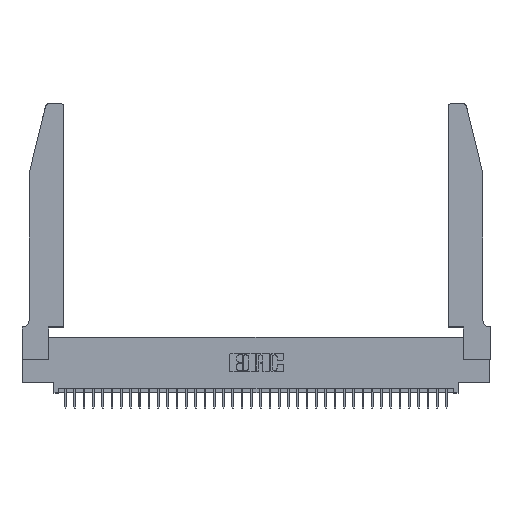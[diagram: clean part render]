
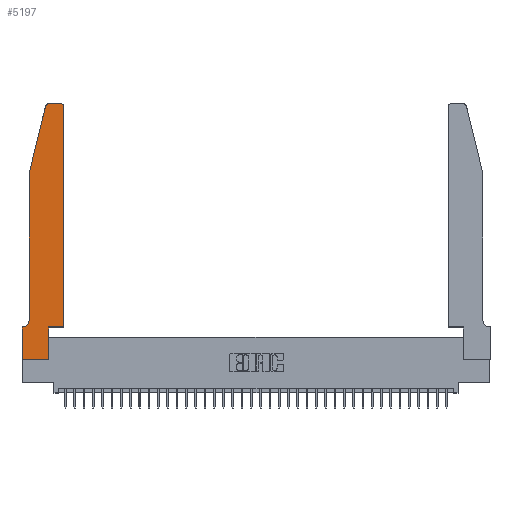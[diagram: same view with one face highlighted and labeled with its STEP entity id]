
A CAD part, top view. The second image highlights one B-rep face of the part: STEP entity #5197.
In plain terms, the highlighted planar face has unit normal (0, 0, 1).
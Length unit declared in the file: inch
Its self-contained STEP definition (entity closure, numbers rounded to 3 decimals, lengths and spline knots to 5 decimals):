
#57 = VECTOR ( 'NONE', #24405, 39.37008 ) ;
#546 = CARTESIAN_POINT ( 'NONE',  ( 0., 0., 0.37 ) ) ;
#634 = LINE ( 'NONE', #9989, #36851 ) ;
#2004 = DIRECTION ( 'NONE',  ( -1., 0., 0. ) ) ;
#2047 = VERTEX_POINT ( 'NONE', #5946 ) ;
#2826 = DIRECTION ( 'NONE',  ( 0., 0., -1. ) ) ;
#4233 = CARTESIAN_POINT ( 'NONE',  ( 0.4505, 0.35, 0.37 ) ) ;
#5197 = ADVANCED_FACE ( 'NONE', ( #11197 ), #16264, .T. ) ;
#5362 = DIRECTION ( 'NONE',  ( 1., 0., 0. ) ) ;
#5784 = AXIS2_PLACEMENT_3D ( 'NONE', #17488, #2826, #16983 ) ;
#5946 = CARTESIAN_POINT ( 'NONE',  ( 0.0755, 0.42, 0.37 ) ) ;
#6552 = DIRECTION ( 'NONE',  ( 0., -1., 0. ) ) ;
#6824 = DIRECTION ( 'NONE',  ( 1., 0., 0. ) ) ;
#6906 = LINE ( 'NONE', #546, #17953 ) ;
#7093 = AXIS2_PLACEMENT_3D ( 'NONE', #24266, #15501, #18473 ) ;
#7154 = VERTEX_POINT ( 'NONE', #23442 ) ;
#7217 = LINE ( 'NONE', #21114, #31999 ) ;
#7551 = DIRECTION ( 'NONE',  ( 0., 1., 0. ) ) ;
#8134 = ORIENTED_EDGE ( 'NONE', *, *, #15051, .T. ) ;
#9388 = LINE ( 'NONE', #19497, #27304 ) ;
#9421 = ORIENTED_EDGE ( 'NONE', *, *, #16220, .T. ) ;
#9503 = CIRCLE ( 'NONE', #32138, 0.03 ) ;
#9526 = DIRECTION ( 'NONE',  ( -0.239, -0.971, 0. ) ) ;
#9819 = ORIENTED_EDGE ( 'NONE', *, *, #16738, .T. ) ;
#9989 = CARTESIAN_POINT ( 'NONE',  ( 0.0755, 2., 0.37 ) ) ;
#10618 = CARTESIAN_POINT ( 'NONE',  ( 0., 0.35, 0.37 ) ) ;
#10877 = VERTEX_POINT ( 'NONE', #31813 ) ;
#11010 = VERTEX_POINT ( 'NONE', #35398 ) ;
#11197 = FACE_OUTER_BOUND ( 'NONE', #14542, .T. ) ;
#11589 = CARTESIAN_POINT ( 'NONE',  ( 0., 0.35, 0.37 ) ) ;
#12143 = CARTESIAN_POINT ( 'NONE',  ( 0., 0., 0.37 ) ) ;
#12635 = LINE ( 'NONE', #17551, #20012 ) ;
#13370 = VERTEX_POINT ( 'NONE', #20096 ) ;
#13848 = CIRCLE ( 'NONE', #5784, 0.07 ) ;
#14542 = EDGE_LOOP ( 'NONE', ( #27543, #8134, #24711, #9819, #24501, #27776, #25364, #32067, #22379, #9421, #22211, #28156 ) ) ;
#14647 = VECTOR ( 'NONE', #24038, 39.37008 ) ;
#14902 = LINE ( 'NONE', #12143, #28696 ) ;
#15051 = EDGE_CURVE ( 'NONE', #24323, #7154, #9503, .T. ) ;
#15501 = DIRECTION ( 'NONE',  ( 0., 0., 1. ) ) ;
#16220 = EDGE_CURVE ( 'NONE', #26213, #26430, #12635, .T. ) ;
#16264 = PLANE ( 'NONE',  #33635 ) ;
#16696 = CARTESIAN_POINT ( 'NONE',  ( 0.284, 2.72, 0.37 ) ) ;
#16702 = CARTESIAN_POINT ( 'NONE',  ( 0.284, 2.75, 0.37 ) ) ;
#16738 = EDGE_CURVE ( 'NONE', #34171, #2047, #634, .T. ) ;
#16983 = DIRECTION ( 'NONE',  ( -1., 0., 0. ) ) ;
#17488 = CARTESIAN_POINT ( 'NONE',  ( 0.0055, 0.42, 0.37 ) ) ;
#17551 = CARTESIAN_POINT ( 'NONE',  ( 0.4505, 0.35, 0.37 ) ) ;
#17953 = VECTOR ( 'NONE', #6824, 39.37008 ) ;
#18473 = DIRECTION ( 'NONE',  ( 1., 0., 0. ) ) ;
#18593 = EDGE_CURVE ( 'NONE', #10877, #11010, #6906, .T. ) ;
#19497 = CARTESIAN_POINT ( 'NONE',  ( 0.0755, 0.35, 0.37 ) ) ;
#19695 = DIRECTION ( 'NONE',  ( 0., 0., 1. ) ) ;
#19731 = EDGE_CURVE ( 'NONE', #33365, #24323, #22490, .T. ) ;
#20012 = VECTOR ( 'NONE', #5362, 39.37008 ) ;
#20096 = CARTESIAN_POINT ( 'NONE',  ( 0.4505, 2.72, 0.37 ) ) ;
#21011 = CARTESIAN_POINT ( 'NONE',  ( 0.2865, 0.35, 0.37 ) ) ;
#21114 = CARTESIAN_POINT ( 'NONE',  ( 0.2865, 0.35, 0.37 ) ) ;
#22211 = ORIENTED_EDGE ( 'NONE', *, *, #24931, .T. ) ;
#22379 = ORIENTED_EDGE ( 'NONE', *, *, #28395, .T. ) ;
#22490 = LINE ( 'NONE', #24155, #14647 ) ;
#23442 = CARTESIAN_POINT ( 'NONE',  ( 0.25487, 2.72718, 0.37 ) ) ;
#23451 = VERTEX_POINT ( 'NONE', #28827 ) ;
#24038 = DIRECTION ( 'NONE',  ( -1., 0., 0. ) ) ;
#24146 = VECTOR ( 'NONE', #9526, 39.37008 ) ;
#24155 = CARTESIAN_POINT ( 'NONE',  ( 0.2605, 2.75, 0.37 ) ) ;
#24266 = CARTESIAN_POINT ( 'NONE',  ( 0.4205, 2.72, 0.37 ) ) ;
#24323 = VERTEX_POINT ( 'NONE', #16702 ) ;
#24405 = DIRECTION ( 'NONE',  ( 0., 1., 0. ) ) ;
#24481 = EDGE_CURVE ( 'NONE', #2047, #23451, #13848, .T. ) ;
#24501 = ORIENTED_EDGE ( 'NONE', *, *, #24481, .T. ) ;
#24711 = ORIENTED_EDGE ( 'NONE', *, *, #29671, .T. ) ;
#24838 = CARTESIAN_POINT ( 'NONE',  ( 0.4205, 2.75, 0.37 ) ) ;
#24931 = EDGE_CURVE ( 'NONE', #26430, #13370, #34942, .T. ) ;
#25364 = ORIENTED_EDGE ( 'NONE', *, *, #34491, .T. ) ;
#26213 = VERTEX_POINT ( 'NONE', #21011 ) ;
#26430 = VERTEX_POINT ( 'NONE', #27939 ) ;
#26855 = CARTESIAN_POINT ( 'NONE',  ( 0.0755, 2., 0.37 ) ) ;
#27304 = VECTOR ( 'NONE', #2004, 39.37008 ) ;
#27543 = ORIENTED_EDGE ( 'NONE', *, *, #19731, .T. ) ;
#27776 = ORIENTED_EDGE ( 'NONE', *, *, #35429, .T. ) ;
#27939 = CARTESIAN_POINT ( 'NONE',  ( 0.4505, 0.35, 0.37 ) ) ;
#28156 = ORIENTED_EDGE ( 'NONE', *, *, #29941, .T. ) ;
#28395 = EDGE_CURVE ( 'NONE', #11010, #26213, #7217, .T. ) ;
#28490 = DIRECTION ( 'NONE',  ( 1., 0., 0. ) ) ;
#28696 = VECTOR ( 'NONE', #32893, 39.37008 ) ;
#28827 = CARTESIAN_POINT ( 'NONE',  ( 0.0055, 0.35, 0.37 ) ) ;
#29671 = EDGE_CURVE ( 'NONE', #7154, #34171, #33722, .T. ) ;
#29941 = EDGE_CURVE ( 'NONE', #13370, #33365, #30126, .T. ) ;
#30126 = CIRCLE ( 'NONE', #7093, 0.03 ) ;
#30882 = DIRECTION ( 'NONE',  ( 0., 0., 1. ) ) ;
#31758 = CARTESIAN_POINT ( 'NONE',  ( 0.0755, 2., 0.37 ) ) ;
#31813 = CARTESIAN_POINT ( 'NONE',  ( 0., 0., 0.37 ) ) ;
#31999 = VECTOR ( 'NONE', #7551, 39.37008 ) ;
#32067 = ORIENTED_EDGE ( 'NONE', *, *, #18593, .T. ) ;
#32138 = AXIS2_PLACEMENT_3D ( 'NONE', #16696, #19695, #37176 ) ;
#32893 = DIRECTION ( 'NONE',  ( 0., -1., 0. ) ) ;
#33365 = VERTEX_POINT ( 'NONE', #24838 ) ;
#33635 = AXIS2_PLACEMENT_3D ( 'NONE', #10618, #30882, #28490 ) ;
#33722 = LINE ( 'NONE', #26855, #24146 ) ;
#34171 = VERTEX_POINT ( 'NONE', #31758 ) ;
#34491 = EDGE_CURVE ( 'NONE', #37863, #10877, #14902, .T. ) ;
#34942 = LINE ( 'NONE', #4233, #57 ) ;
#35398 = CARTESIAN_POINT ( 'NONE',  ( 0.2865, 0., 0.37 ) ) ;
#35429 = EDGE_CURVE ( 'NONE', #23451, #37863, #9388, .T. ) ;
#36851 = VECTOR ( 'NONE', #6552, 39.37008 ) ;
#37176 = DIRECTION ( 'NONE',  ( 1., 0., 0. ) ) ;
#37863 = VERTEX_POINT ( 'NONE', #11589 ) ;
